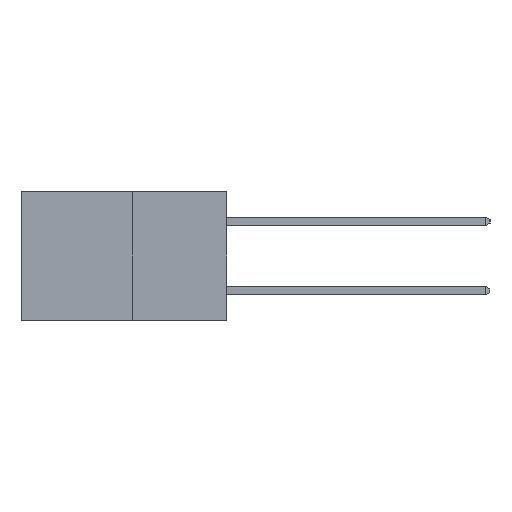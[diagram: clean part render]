
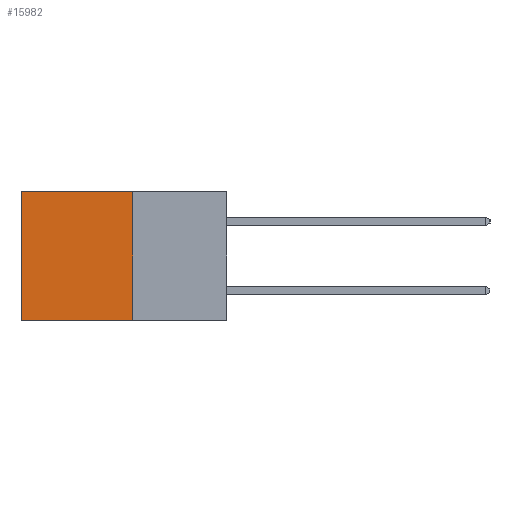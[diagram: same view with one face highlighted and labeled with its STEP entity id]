
A CAD part, left-side view. The second image highlights one B-rep face of the part: STEP entity #15982.
In plain terms, the highlighted planar face has unit normal (-1, 0, 0).
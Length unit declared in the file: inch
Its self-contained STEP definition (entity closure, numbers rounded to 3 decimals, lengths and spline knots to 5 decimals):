
#142 = CARTESIAN_POINT ( 'NONE',  ( 0.277, 0.59, 0. ) ) ;
#1468 = CARTESIAN_POINT ( 'NONE',  ( 0.277, 0.27, -0.37 ) ) ;
#1569 = LINE ( 'NONE', #16160, #13367 ) ;
#1946 = CARTESIAN_POINT ( 'NONE',  ( 0.277, 0.27, -0.37 ) ) ;
#2662 = ORIENTED_EDGE ( 'NONE', *, *, #2670, .T. ) ;
#2670 = EDGE_CURVE ( 'NONE', #13894, #19039, #11364, .T. ) ;
#3634 = DIRECTION ( 'NONE',  ( 0., 0., -1. ) ) ;
#4576 = ORIENTED_EDGE ( 'NONE', *, *, #14741, .F. ) ;
#5223 = VECTOR ( 'NONE', #18134, 39.37008 ) ;
#5749 = EDGE_LOOP ( 'NONE', ( #2662, #12504, #4576, #18656 ) ) ;
#8200 = AXIS2_PLACEMENT_3D ( 'NONE', #1946, #13154, #3634 ) ;
#8977 = CARTESIAN_POINT ( 'NONE',  ( 0.277, 0.27, -0.37 ) ) ;
#9122 = EDGE_CURVE ( 'NONE', #12306, #19039, #10412, .T. ) ;
#10299 = LINE ( 'NONE', #11721, #14936 ) ;
#10336 = CARTESIAN_POINT ( 'NONE',  ( 0.277, 0.27, 0. ) ) ;
#10412 = LINE ( 'NONE', #8977, #5223 ) ;
#11364 = LINE ( 'NONE', #12033, #14997 ) ;
#11577 = EDGE_CURVE ( 'NONE', #12660, #13894, #1569, .T. ) ;
#11721 = CARTESIAN_POINT ( 'NONE',  ( 0.277, 0.27, -0.37 ) ) ;
#12033 = CARTESIAN_POINT ( 'NONE',  ( 0.277, 0.59, -0.37 ) ) ;
#12306 = VERTEX_POINT ( 'NONE', #1468 ) ;
#12504 = ORIENTED_EDGE ( 'NONE', *, *, #9122, .F. ) ;
#12660 = VERTEX_POINT ( 'NONE', #10336 ) ;
#13154 = DIRECTION ( 'NONE',  ( 1., 0., 0. ) ) ;
#13367 = VECTOR ( 'NONE', #17660, 39.37008 ) ;
#13894 = VERTEX_POINT ( 'NONE', #142 ) ;
#14741 = EDGE_CURVE ( 'NONE', #12660, #12306, #10299, .T. ) ;
#14936 = VECTOR ( 'NONE', #19268, 39.37008 ) ;
#14997 = VECTOR ( 'NONE', #16976, 39.37008 ) ;
#15441 = FACE_OUTER_BOUND ( 'NONE', #5749, .T. ) ;
#15982 = ADVANCED_FACE ( 'NONE', ( #15441 ), #17601, .F. ) ;
#16160 = CARTESIAN_POINT ( 'NONE',  ( 0.277, 0.27, 0. ) ) ;
#16518 = CARTESIAN_POINT ( 'NONE',  ( 0.277, 0.59, -0.37 ) ) ;
#16976 = DIRECTION ( 'NONE',  ( 0., 0., -1. ) ) ;
#17601 = PLANE ( 'NONE',  #8200 ) ;
#17660 = DIRECTION ( 'NONE',  ( 0., 1., 0. ) ) ;
#18134 = DIRECTION ( 'NONE',  ( 0., 1., 0. ) ) ;
#18656 = ORIENTED_EDGE ( 'NONE', *, *, #11577, .T. ) ;
#19039 = VERTEX_POINT ( 'NONE', #16518 ) ;
#19268 = DIRECTION ( 'NONE',  ( 0., 0., -1. ) ) ;
